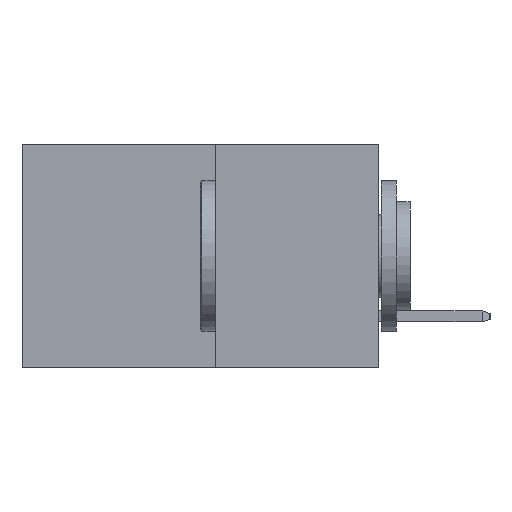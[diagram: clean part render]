
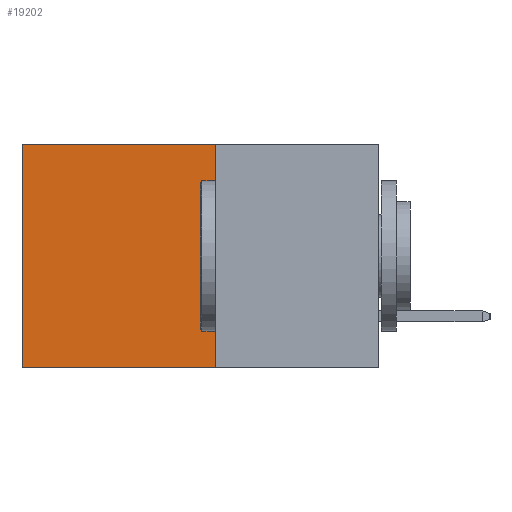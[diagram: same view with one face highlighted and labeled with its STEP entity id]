
A CAD part, left-side view. The second image highlights one B-rep face of the part: STEP entity #19202.
In plain terms, the highlighted planar face has unit normal (-1, 0, 0).
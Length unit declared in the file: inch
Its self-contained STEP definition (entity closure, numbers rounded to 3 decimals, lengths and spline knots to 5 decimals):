
#1476 = VECTOR ( 'NONE', #5552, 39.37008 ) ;
#1547 = CARTESIAN_POINT ( 'NONE',  ( 0.277, 0.27, -0.37 ) ) ;
#2407 = FACE_OUTER_BOUND ( 'NONE', #15888, .T. ) ;
#2742 = VECTOR ( 'NONE', #3571, 39.37008 ) ;
#3571 = DIRECTION ( 'NONE',  ( 0., 1., 0. ) ) ;
#3842 = CARTESIAN_POINT ( 'NONE',  ( 0.277, 0.27, 0. ) ) ;
#4002 = LINE ( 'NONE', #5515, #17909 ) ;
#4519 = EDGE_CURVE ( 'NONE', #11827, #21279, #12083, .T. ) ;
#5515 = CARTESIAN_POINT ( 'NONE',  ( 0.277, 0.59, -0.37 ) ) ;
#5552 = DIRECTION ( 'NONE',  ( 0., 0., -1. ) ) ;
#6023 = CARTESIAN_POINT ( 'NONE',  ( 0.277, 0.27, -0.37 ) ) ;
#6306 = EDGE_CURVE ( 'NONE', #11827, #8501, #24323, .T. ) ;
#7946 = DIRECTION ( 'NONE',  ( 1., 0., 0. ) ) ;
#8501 = VERTEX_POINT ( 'NONE', #16320 ) ;
#9230 = DIRECTION ( 'NONE',  ( 0., 1., 0. ) ) ;
#9619 = CARTESIAN_POINT ( 'NONE',  ( 0.277, 0.27, 0. ) ) ;
#10064 = CARTESIAN_POINT ( 'NONE',  ( 0.277, 0.27, -0.37 ) ) ;
#11827 = VERTEX_POINT ( 'NONE', #3842 ) ;
#12083 = LINE ( 'NONE', #6023, #1476 ) ;
#12697 = ORIENTED_EDGE ( 'NONE', *, *, #4519, .F. ) ;
#12822 = ORIENTED_EDGE ( 'NONE', *, *, #23319, .F. ) ;
#13208 = AXIS2_PLACEMENT_3D ( 'NONE', #17717, #7946, #21542 ) ;
#13771 = PLANE ( 'NONE',  #13208 ) ;
#13908 = ORIENTED_EDGE ( 'NONE', *, *, #6306, .T. ) ;
#14158 = VECTOR ( 'NONE', #9230, 39.37008 ) ;
#15888 = EDGE_LOOP ( 'NONE', ( #19858, #12822, #12697, #13908 ) ) ;
#16320 = CARTESIAN_POINT ( 'NONE',  ( 0.277, 0.59, 0. ) ) ;
#17717 = CARTESIAN_POINT ( 'NONE',  ( 0.277, 0.27, -0.37 ) ) ;
#17765 = CARTESIAN_POINT ( 'NONE',  ( 0.277, 0.59, -0.37 ) ) ;
#17909 = VECTOR ( 'NONE', #19341, 39.37008 ) ;
#18510 = LINE ( 'NONE', #1547, #2742 ) ;
#19202 = ADVANCED_FACE ( 'NONE', ( #2407 ), #13771, .F. ) ;
#19341 = DIRECTION ( 'NONE',  ( 0., 0., -1. ) ) ;
#19858 = ORIENTED_EDGE ( 'NONE', *, *, #23341, .T. ) ;
#19969 = VERTEX_POINT ( 'NONE', #17765 ) ;
#21279 = VERTEX_POINT ( 'NONE', #10064 ) ;
#21542 = DIRECTION ( 'NONE',  ( 0., 0., -1. ) ) ;
#23319 = EDGE_CURVE ( 'NONE', #21279, #19969, #18510, .T. ) ;
#23341 = EDGE_CURVE ( 'NONE', #8501, #19969, #4002, .T. ) ;
#24323 = LINE ( 'NONE', #9619, #14158 ) ;
